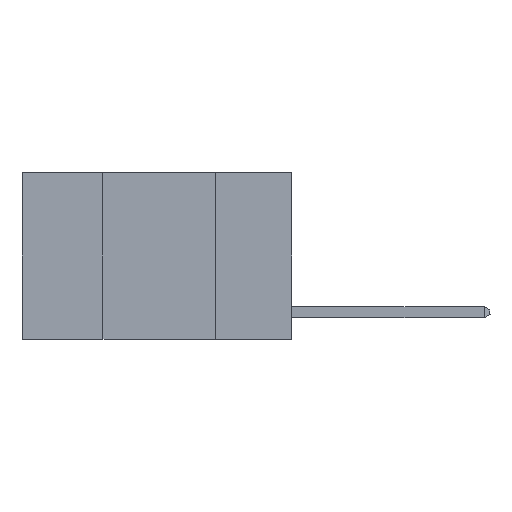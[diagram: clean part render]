
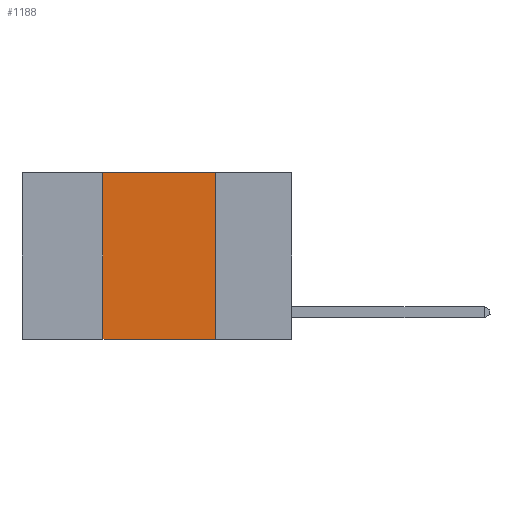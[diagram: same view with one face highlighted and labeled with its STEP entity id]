
A CAD part, left-side view. The second image highlights one B-rep face of the part: STEP entity #1188.
In plain terms, the highlighted planar face has unit normal (-1, 0, 0).
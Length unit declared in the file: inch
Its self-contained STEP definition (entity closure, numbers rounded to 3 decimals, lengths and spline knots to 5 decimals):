
#631 = CARTESIAN_POINT ( 'NONE',  ( 0., 0.17, 0. ) ) ;
#703 = DIRECTION ( 'NONE',  ( 0., 0., 1. ) ) ;
#932 = VERTEX_POINT ( 'NONE', #9468 ) ;
#1188 = ADVANCED_FACE ( 'NONE', ( #9346 ), #1950, .F. ) ;
#1518 = LINE ( 'NONE', #5271, #4519 ) ;
#1568 = DIRECTION ( 'NONE',  ( 0., -1., 0. ) ) ;
#1950 = PLANE ( 'NONE',  #8489 ) ;
#2329 = VERTEX_POINT ( 'NONE', #7383 ) ;
#2741 = VERTEX_POINT ( 'NONE', #7405 ) ;
#2804 = VECTOR ( 'NONE', #2835, 39.37008 ) ;
#2835 = DIRECTION ( 'NONE',  ( 0., 0., -1. ) ) ;
#3881 = EDGE_CURVE ( 'NONE', #2741, #2329, #5644, .T. ) ;
#4104 = VECTOR ( 'NONE', #703, 39.37008 ) ;
#4224 = VERTEX_POINT ( 'NONE', #8878 ) ;
#4378 = LINE ( 'NONE', #7350, #4104 ) ;
#4519 = VECTOR ( 'NONE', #1568, 39.37008 ) ;
#4869 = CARTESIAN_POINT ( 'NONE',  ( 0., 0.6, 0. ) ) ;
#4953 = DIRECTION ( 'NONE',  ( 0., -1., 0. ) ) ;
#5271 = CARTESIAN_POINT ( 'NONE',  ( 0., 0.6, 0. ) ) ;
#5302 = EDGE_CURVE ( 'NONE', #2741, #932, #4378, .T. ) ;
#5489 = ORIENTED_EDGE ( 'NONE', *, *, #7321, .F. ) ;
#5586 = EDGE_LOOP ( 'NONE', ( #8951, #5489, #9199, #9081 ) ) ;
#5644 = LINE ( 'NONE', #8668, #6390 ) ;
#6390 = VECTOR ( 'NONE', #4953, 39.37008 ) ;
#7125 = DIRECTION ( 'NONE',  ( 0., 0., -1. ) ) ;
#7321 = EDGE_CURVE ( 'NONE', #932, #4224, #1518, .T. ) ;
#7350 = CARTESIAN_POINT ( 'NONE',  ( 0., 0.42, 0. ) ) ;
#7383 = CARTESIAN_POINT ( 'NONE',  ( 0., 0.17, -0.37 ) ) ;
#7405 = CARTESIAN_POINT ( 'NONE',  ( 0., 0.42, -0.37 ) ) ;
#7915 = DIRECTION ( 'NONE',  ( 1., 0., 0. ) ) ;
#8004 = EDGE_CURVE ( 'NONE', #4224, #2329, #9473, .T. ) ;
#8489 = AXIS2_PLACEMENT_3D ( 'NONE', #4869, #7915, #7125 ) ;
#8668 = CARTESIAN_POINT ( 'NONE',  ( 0., 0.6, -0.37 ) ) ;
#8878 = CARTESIAN_POINT ( 'NONE',  ( 0., 0.17, 0. ) ) ;
#8951 = ORIENTED_EDGE ( 'NONE', *, *, #8004, .F. ) ;
#9081 = ORIENTED_EDGE ( 'NONE', *, *, #3881, .T. ) ;
#9199 = ORIENTED_EDGE ( 'NONE', *, *, #5302, .F. ) ;
#9346 = FACE_OUTER_BOUND ( 'NONE', #5586, .T. ) ;
#9468 = CARTESIAN_POINT ( 'NONE',  ( 0., 0.42, 0. ) ) ;
#9473 = LINE ( 'NONE', #631, #2804 ) ;
